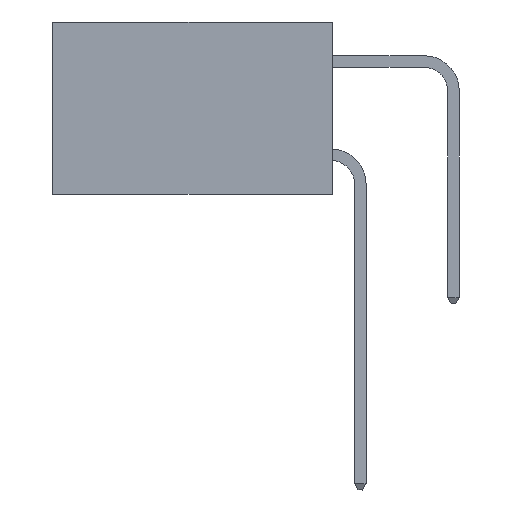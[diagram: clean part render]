
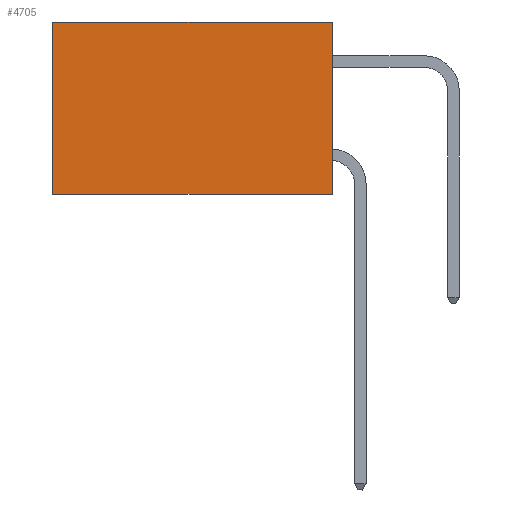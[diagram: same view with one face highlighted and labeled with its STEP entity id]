
A CAD part, left-side view. The second image highlights one B-rep face of the part: STEP entity #4705.
In plain terms, the highlighted planar face has unit normal (-1, 0, 0).
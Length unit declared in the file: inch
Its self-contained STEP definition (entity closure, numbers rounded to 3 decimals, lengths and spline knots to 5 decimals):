
#728 = CARTESIAN_POINT ( 'NONE',  ( 0.298, 0.6, -0.37 ) ) ;
#973 = CARTESIAN_POINT ( 'NONE',  ( 0.298, 0., -0.37 ) ) ;
#1329 = LINE ( 'NONE', #5356, #4431 ) ;
#1621 = EDGE_CURVE ( 'NONE', #6969, #1626, #2393, .T. ) ;
#1626 = VERTEX_POINT ( 'NONE', #728 ) ;
#2393 = LINE ( 'NONE', #973, #10566 ) ;
#3162 = CARTESIAN_POINT ( 'NONE',  ( 0.298, 0., 0. ) ) ;
#3345 = VECTOR ( 'NONE', #11635, 39.37008 ) ;
#3791 = DIRECTION ( 'NONE',  ( 0., 1., 0. ) ) ;
#4431 = VECTOR ( 'NONE', #7393, 39.37008 ) ;
#4475 = FACE_OUTER_BOUND ( 'NONE', #6466, .T. ) ;
#4705 = ADVANCED_FACE ( 'NONE', ( #4475 ), #9947, .F. ) ;
#5142 = DIRECTION ( 'NONE',  ( 0., 0., -1. ) ) ;
#5226 = ORIENTED_EDGE ( 'NONE', *, *, #10993, .F. ) ;
#5356 = CARTESIAN_POINT ( 'NONE',  ( 0.298, 0.6, 0. ) ) ;
#5867 = ORIENTED_EDGE ( 'NONE', *, *, #9296, .T. ) ;
#5976 = CARTESIAN_POINT ( 'NONE',  ( 0.298, 0., 0. ) ) ;
#6466 = EDGE_LOOP ( 'NONE', ( #12545, #12330, #5226, #5867 ) ) ;
#6969 = VERTEX_POINT ( 'NONE', #10954 ) ;
#7393 = DIRECTION ( 'NONE',  ( 0., 0., -1. ) ) ;
#7459 = LINE ( 'NONE', #11413, #11404 ) ;
#8436 = VERTEX_POINT ( 'NONE', #5976 ) ;
#8597 = LINE ( 'NONE', #8672, #3345 ) ;
#8672 = CARTESIAN_POINT ( 'NONE',  ( 0.298, 0., 0. ) ) ;
#9296 = EDGE_CURVE ( 'NONE', #8436, #9732, #7459, .T. ) ;
#9382 = CARTESIAN_POINT ( 'NONE',  ( 0.298, 0.6, 0. ) ) ;
#9386 = AXIS2_PLACEMENT_3D ( 'NONE', #3162, #10932, #5142 ) ;
#9732 = VERTEX_POINT ( 'NONE', #9382 ) ;
#9947 = PLANE ( 'NONE',  #9386 ) ;
#10203 = EDGE_CURVE ( 'NONE', #9732, #1626, #1329, .T. ) ;
#10421 = DIRECTION ( 'NONE',  ( 0., 1., 0. ) ) ;
#10566 = VECTOR ( 'NONE', #3791, 39.37008 ) ;
#10932 = DIRECTION ( 'NONE',  ( 1., 0., 0. ) ) ;
#10954 = CARTESIAN_POINT ( 'NONE',  ( 0.298, 0., -0.37 ) ) ;
#10993 = EDGE_CURVE ( 'NONE', #8436, #6969, #8597, .T. ) ;
#11404 = VECTOR ( 'NONE', #10421, 39.37008 ) ;
#11413 = CARTESIAN_POINT ( 'NONE',  ( 0.298, 0., 0. ) ) ;
#11635 = DIRECTION ( 'NONE',  ( 0., 0., -1. ) ) ;
#12330 = ORIENTED_EDGE ( 'NONE', *, *, #1621, .F. ) ;
#12545 = ORIENTED_EDGE ( 'NONE', *, *, #10203, .T. ) ;
